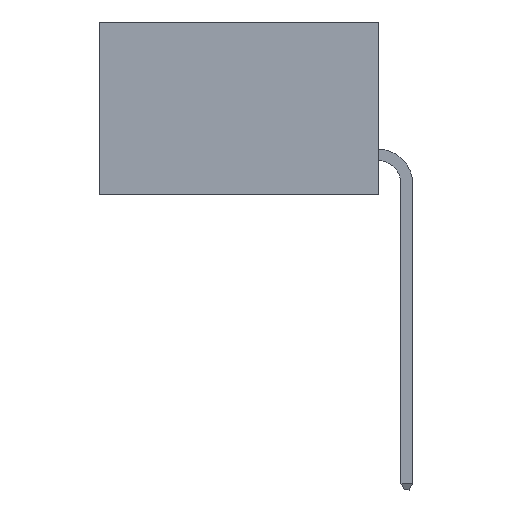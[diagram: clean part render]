
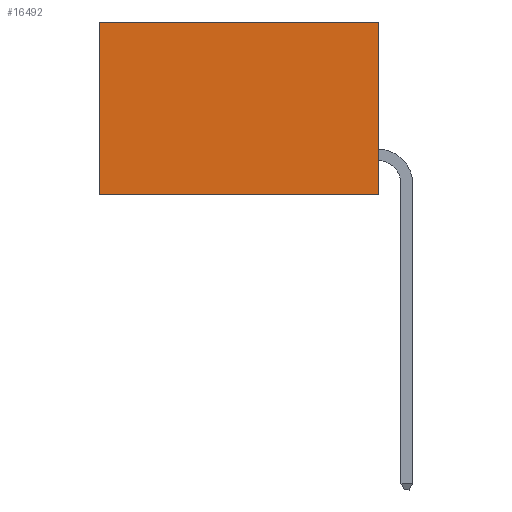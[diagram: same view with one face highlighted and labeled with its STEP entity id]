
A CAD part, left-side view. The second image highlights one B-rep face of the part: STEP entity #16492.
In plain terms, the highlighted planar face has unit normal (-1, 0, 0).
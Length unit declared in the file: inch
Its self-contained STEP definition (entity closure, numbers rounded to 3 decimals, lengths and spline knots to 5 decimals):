
#396 = CARTESIAN_POINT ( 'NONE',  ( 0.298, 0., 0. ) ) ;
#707 = FACE_OUTER_BOUND ( 'NONE', #10548, .T. ) ;
#1465 = VECTOR ( 'NONE', #15074, 39.37008 ) ;
#1679 = CARTESIAN_POINT ( 'NONE',  ( 0.298, 0., -0.37 ) ) ;
#2289 = VECTOR ( 'NONE', #3485, 39.37008 ) ;
#2471 = VERTEX_POINT ( 'NONE', #6790 ) ;
#3485 = DIRECTION ( 'NONE',  ( 0., 0., -1. ) ) ;
#5049 = EDGE_CURVE ( 'NONE', #23477, #26177, #18929, .T. ) ;
#5999 = VERTEX_POINT ( 'NONE', #20750 ) ;
#6507 = ORIENTED_EDGE ( 'NONE', *, *, #5049, .F. ) ;
#6790 = CARTESIAN_POINT ( 'NONE',  ( 0.298, 0.6, -0.37 ) ) ;
#8104 = LINE ( 'NONE', #18795, #2289 ) ;
#8539 = DIRECTION ( 'NONE',  ( 0., 0., -1. ) ) ;
#10037 = ORIENTED_EDGE ( 'NONE', *, *, #26707, .T. ) ;
#10548 = EDGE_LOOP ( 'NONE', ( #10037, #13747, #6507, #25042 ) ) ;
#13490 = LINE ( 'NONE', #15945, #18610 ) ;
#13747 = ORIENTED_EDGE ( 'NONE', *, *, #15374, .F. ) ;
#14166 = CARTESIAN_POINT ( 'NONE',  ( 0.298, 0., 0. ) ) ;
#15074 = DIRECTION ( 'NONE',  ( 0., 0., -1. ) ) ;
#15259 = AXIS2_PLACEMENT_3D ( 'NONE', #25714, #21573, #8539 ) ;
#15374 = EDGE_CURVE ( 'NONE', #26177, #2471, #13490, .T. ) ;
#15460 = VECTOR ( 'NONE', #21839, 39.37008 ) ;
#15945 = CARTESIAN_POINT ( 'NONE',  ( 0.298, 0., -0.37 ) ) ;
#16492 = ADVANCED_FACE ( 'NONE', ( #707 ), #19411, .F. ) ;
#16575 = EDGE_CURVE ( 'NONE', #23477, #5999, #26737, .T. ) ;
#18105 = DIRECTION ( 'NONE',  ( 0., 1., 0. ) ) ;
#18610 = VECTOR ( 'NONE', #18105, 39.37008 ) ;
#18795 = CARTESIAN_POINT ( 'NONE',  ( 0.298, 0.6, 0. ) ) ;
#18929 = LINE ( 'NONE', #396, #1465 ) ;
#19411 = PLANE ( 'NONE',  #15259 ) ;
#20750 = CARTESIAN_POINT ( 'NONE',  ( 0.298, 0.6, 0. ) ) ;
#21573 = DIRECTION ( 'NONE',  ( 1., 0., 0. ) ) ;
#21839 = DIRECTION ( 'NONE',  ( 0., 1., 0. ) ) ;
#23477 = VERTEX_POINT ( 'NONE', #14166 ) ;
#25042 = ORIENTED_EDGE ( 'NONE', *, *, #16575, .T. ) ;
#25714 = CARTESIAN_POINT ( 'NONE',  ( 0.298, 0., 0. ) ) ;
#25972 = CARTESIAN_POINT ( 'NONE',  ( 0.298, 0., 0. ) ) ;
#26177 = VERTEX_POINT ( 'NONE', #1679 ) ;
#26707 = EDGE_CURVE ( 'NONE', #5999, #2471, #8104, .T. ) ;
#26737 = LINE ( 'NONE', #25972, #15460 ) ;
